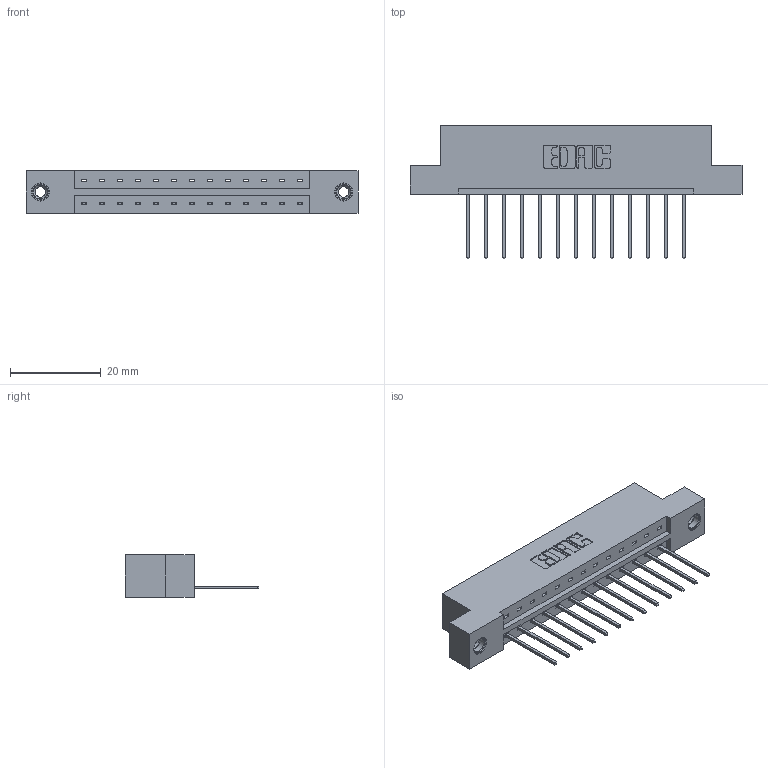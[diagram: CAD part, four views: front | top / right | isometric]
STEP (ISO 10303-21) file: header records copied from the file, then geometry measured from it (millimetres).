
FILE_DESCRIPTION (( 'STEP AP203' ), '1' );
FILE_NAME ('833-013-540-108.STEP', '2020-05-31T00:00:34', ( '' ), ( '' ), 'SwSTEP 2.0', 'SolidWorks 2020', '' );
FILE_SCHEMA (( 'CONFIG_CONTROL_DESIGN' ));
Length unit declared in the file: inch
Products named in the file (4): 833-013-540-108; 345-250-001_345-250-003-102; 833 Part_Flush - .156 Dia - TI; 345-292-001_345-293-140
Assembly tree (16 placements, depth 2):
  833-013-540-108
    833 Part_Flush - .156 Dia - TI
    345-292-001_345-293-140  x13
    345-250-001_345-250-003-102  x2
Bounding box: 73.05 x 29.47 x 9.4 mm (x, y, z)
Volume: 7112.6 mm3; surface area: 7663.2 mm2
Topology: 16 solids, 16 shells, 928 faces, 2735 edges, 1798 vertices
Faces by surface type: plane 648, cylinder 264, cone 12, torus 4
Entity records: 12902 total; most frequent: CARTESIAN_POINT 2212, ORIENTED_EDGE 2154, DIRECTION 1957, EDGE_CURVE 1077, VECTOR 929, LINE 929, VERTEX_POINT 712, AXIS2_PLACEMENT_3D 514
